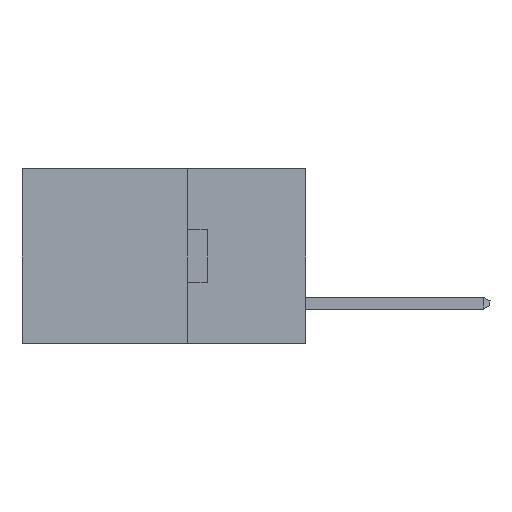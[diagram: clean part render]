
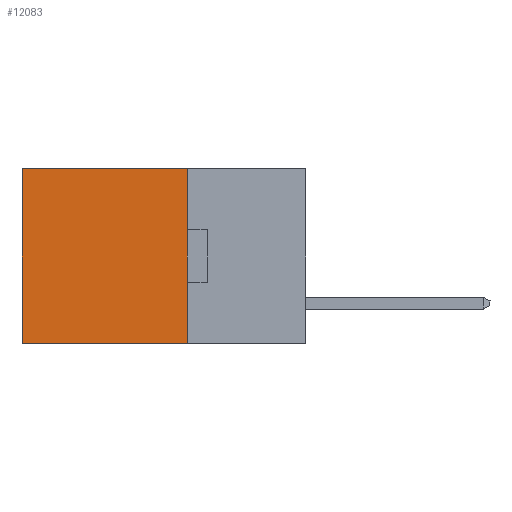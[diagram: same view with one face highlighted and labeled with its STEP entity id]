
A CAD part, left-side view. The second image highlights one B-rep face of the part: STEP entity #12083.
In plain terms, the highlighted planar face has unit normal (-1, 0, 0).
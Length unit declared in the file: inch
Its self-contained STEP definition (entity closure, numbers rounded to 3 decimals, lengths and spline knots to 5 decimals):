
#99 = ORIENTED_EDGE ( 'NONE', *, *, #5478, .F. ) ;
#860 = PLANE ( 'NONE',  #18335 ) ;
#3075 = DIRECTION ( 'NONE',  ( 0., 0., -1. ) ) ;
#3401 = CARTESIAN_POINT ( 'NONE',  ( 0.2615, 0.6, -0.37 ) ) ;
#3837 = CARTESIAN_POINT ( 'NONE',  ( 0.2615, 0.25, 0. ) ) ;
#5115 = CARTESIAN_POINT ( 'NONE',  ( 0.2615, 0.25, -0.37 ) ) ;
#5478 = EDGE_CURVE ( 'NONE', #15479, #9911, #5649, .T. ) ;
#5649 = LINE ( 'NONE', #5115, #20354 ) ;
#5825 = DIRECTION ( 'NONE',  ( 0., 0., -1. ) ) ;
#7237 = DIRECTION ( 'NONE',  ( 1., 0., 0. ) ) ;
#8576 = EDGE_CURVE ( 'NONE', #9640, #23800, #16574, .T. ) ;
#9634 = EDGE_CURVE ( 'NONE', #9640, #15479, #13859, .T. ) ;
#9640 = VERTEX_POINT ( 'NONE', #20523 ) ;
#9911 = VERTEX_POINT ( 'NONE', #3401 ) ;
#9966 = CARTESIAN_POINT ( 'NONE',  ( 0.2615, 0.25, -0.37 ) ) ;
#10066 = DIRECTION ( 'NONE',  ( 0., 1., 0. ) ) ;
#11653 = FACE_OUTER_BOUND ( 'NONE', #23351, .T. ) ;
#12050 = VECTOR ( 'NONE', #10066, 39.37008 ) ;
#12071 = ORIENTED_EDGE ( 'NONE', *, *, #9634, .F. ) ;
#12083 = ADVANCED_FACE ( 'NONE', ( #11653 ), #860, .F. ) ;
#12110 = VECTOR ( 'NONE', #16746, 39.37008 ) ;
#12192 = EDGE_CURVE ( 'NONE', #23800, #9911, #27280, .T. ) ;
#13851 = VECTOR ( 'NONE', #5825, 39.37008 ) ;
#13859 = LINE ( 'NONE', #9966, #13851 ) ;
#13972 = CARTESIAN_POINT ( 'NONE',  ( 0.2615, 0.6, 0. ) ) ;
#15394 = ORIENTED_EDGE ( 'NONE', *, *, #8576, .T. ) ;
#15479 = VERTEX_POINT ( 'NONE', #15767 ) ;
#15767 = CARTESIAN_POINT ( 'NONE',  ( 0.2615, 0.25, -0.37 ) ) ;
#16349 = CARTESIAN_POINT ( 'NONE',  ( 0.2615, 0.6, -0.37 ) ) ;
#16574 = LINE ( 'NONE', #3837, #12050 ) ;
#16746 = DIRECTION ( 'NONE',  ( 0., 0., -1. ) ) ;
#18335 = AXIS2_PLACEMENT_3D ( 'NONE', #26344, #7237, #3075 ) ;
#19129 = ORIENTED_EDGE ( 'NONE', *, *, #12192, .T. ) ;
#20210 = DIRECTION ( 'NONE',  ( 0., 1., 0. ) ) ;
#20354 = VECTOR ( 'NONE', #20210, 39.37008 ) ;
#20523 = CARTESIAN_POINT ( 'NONE',  ( 0.2615, 0.25, 0. ) ) ;
#23351 = EDGE_LOOP ( 'NONE', ( #19129, #99, #12071, #15394 ) ) ;
#23800 = VERTEX_POINT ( 'NONE', #13972 ) ;
#26344 = CARTESIAN_POINT ( 'NONE',  ( 0.2615, 0.25, -0.37 ) ) ;
#27280 = LINE ( 'NONE', #16349, #12110 ) ;
